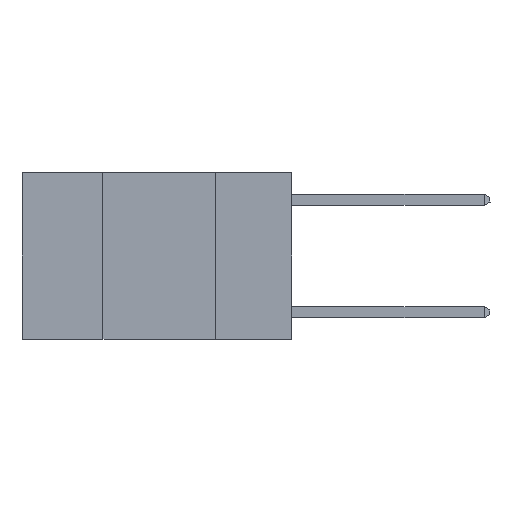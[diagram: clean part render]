
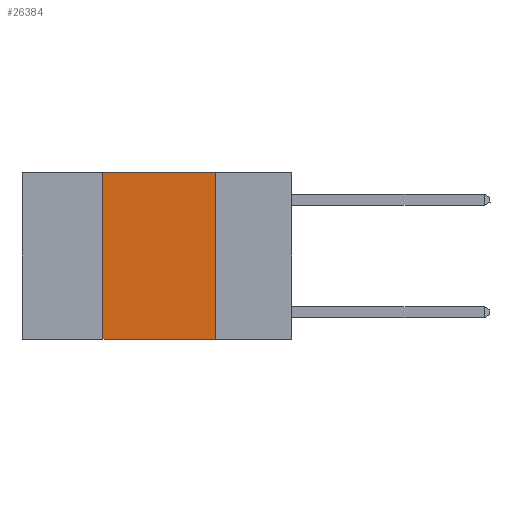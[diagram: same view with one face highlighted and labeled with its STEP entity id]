
A CAD part, left-side view. The second image highlights one B-rep face of the part: STEP entity #26384.
In plain terms, the highlighted planar face has unit normal (-1, 0, 0).
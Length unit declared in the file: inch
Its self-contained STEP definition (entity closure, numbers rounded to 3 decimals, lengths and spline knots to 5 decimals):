
#701 = FACE_OUTER_BOUND ( 'NONE', #15732, .T. ) ;
#1167 = DIRECTION ( 'NONE',  ( 0., 0., -1. ) ) ;
#4357 = DIRECTION ( 'NONE',  ( 0., 0., 1. ) ) ;
#4515 = ORIENTED_EDGE ( 'NONE', *, *, #26563, .F. ) ;
#6736 = VECTOR ( 'NONE', #28859, 39.37008 ) ;
#6790 = CARTESIAN_POINT ( 'NONE',  ( 0., 0.6, -0.37 ) ) ;
#7452 = DIRECTION ( 'NONE',  ( 0., -1., 0. ) ) ;
#7951 = VERTEX_POINT ( 'NONE', #13690 ) ;
#8441 = VECTOR ( 'NONE', #4357, 39.37008 ) ;
#8873 = LINE ( 'NONE', #11951, #20503 ) ;
#9526 = DIRECTION ( 'NONE',  ( 0., 0., -1. ) ) ;
#11407 = AXIS2_PLACEMENT_3D ( 'NONE', #13547, #15999, #1167 ) ;
#11820 = EDGE_CURVE ( 'NONE', #25395, #7951, #19882, .T. ) ;
#11951 = CARTESIAN_POINT ( 'NONE',  ( 0., 0.17, 0. ) ) ;
#13547 = CARTESIAN_POINT ( 'NONE',  ( 0., 0.6, 0. ) ) ;
#13690 = CARTESIAN_POINT ( 'NONE',  ( 0., 0.17, -0.37 ) ) ;
#15118 = ORIENTED_EDGE ( 'NONE', *, *, #11820, .T. ) ;
#15732 = EDGE_LOOP ( 'NONE', ( #24978, #30937, #4515, #15118 ) ) ;
#15999 = DIRECTION ( 'NONE',  ( 1., 0., 0. ) ) ;
#17050 = VECTOR ( 'NONE', #7452, 39.37008 ) ;
#17287 = CARTESIAN_POINT ( 'NONE',  ( 0., 0.6, 0. ) ) ;
#19882 = LINE ( 'NONE', #6790, #6736 ) ;
#20503 = VECTOR ( 'NONE', #9526, 39.37008 ) ;
#21586 = CARTESIAN_POINT ( 'NONE',  ( 0., 0.42, 0. ) ) ;
#21605 = EDGE_CURVE ( 'NONE', #29361, #24415, #24338, .T. ) ;
#22091 = CARTESIAN_POINT ( 'NONE',  ( 0., 0.42, -0.37 ) ) ;
#22870 = EDGE_CURVE ( 'NONE', #24415, #7951, #8873, .T. ) ;
#24338 = LINE ( 'NONE', #17287, #17050 ) ;
#24415 = VERTEX_POINT ( 'NONE', #27941 ) ;
#24978 = ORIENTED_EDGE ( 'NONE', *, *, #22870, .F. ) ;
#25395 = VERTEX_POINT ( 'NONE', #22091 ) ;
#25845 = CARTESIAN_POINT ( 'NONE',  ( 0., 0.42, 0. ) ) ;
#26384 = ADVANCED_FACE ( 'NONE', ( #701 ), #30557, .F. ) ;
#26563 = EDGE_CURVE ( 'NONE', #25395, #29361, #27245, .T. ) ;
#27245 = LINE ( 'NONE', #21586, #8441 ) ;
#27941 = CARTESIAN_POINT ( 'NONE',  ( 0., 0.17, 0. ) ) ;
#28859 = DIRECTION ( 'NONE',  ( 0., -1., 0. ) ) ;
#29361 = VERTEX_POINT ( 'NONE', #25845 ) ;
#30557 = PLANE ( 'NONE',  #11407 ) ;
#30937 = ORIENTED_EDGE ( 'NONE', *, *, #21605, .F. ) ;
